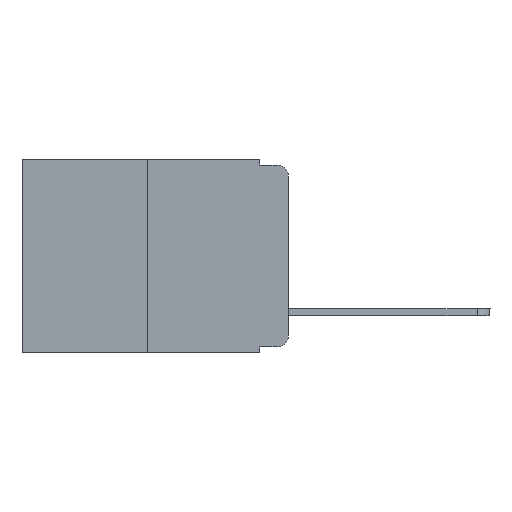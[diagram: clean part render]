
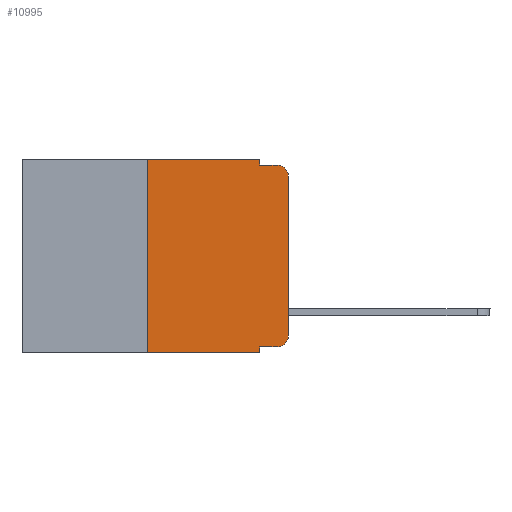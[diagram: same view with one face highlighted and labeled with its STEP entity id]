
A CAD part, left-side view. The second image highlights one B-rep face of the part: STEP entity #10995.
In plain terms, the highlighted planar face has unit normal (-1, 0, 0).
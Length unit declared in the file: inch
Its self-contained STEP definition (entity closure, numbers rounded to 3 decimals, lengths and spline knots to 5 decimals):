
#72 = ORIENTED_EDGE ( 'NONE', *, *, #10749, .T. ) ;
#317 = CARTESIAN_POINT ( 'NONE',  ( 0., 0.051, -0.01 ) ) ;
#686 = CIRCLE ( 'NONE', #3848, 0.02 ) ;
#906 = ORIENTED_EDGE ( 'NONE', *, *, #10365, .T. ) ;
#1024 = CARTESIAN_POINT ( 'NONE',  ( 0., 0.051, -0.01 ) ) ;
#1031 = VECTOR ( 'NONE', #2247, 39.37008 ) ;
#1064 = CARTESIAN_POINT ( 'NONE',  ( 0., 0., -0.313 ) ) ;
#1391 = FACE_OUTER_BOUND ( 'NONE', #3093, .T. ) ;
#1834 = EDGE_CURVE ( 'NONE', #2476, #7793, #9670, .T. ) ;
#1972 = DIRECTION ( 'NONE',  ( 0., 0., 1. ) ) ;
#2091 = CARTESIAN_POINT ( 'NONE',  ( 0., 0.051, -0.333 ) ) ;
#2111 = LINE ( 'NONE', #15091, #1031 ) ;
#2233 = VERTEX_POINT ( 'NONE', #2091 ) ;
#2247 = DIRECTION ( 'NONE',  ( 0., -1., 0. ) ) ;
#2476 = VERTEX_POINT ( 'NONE', #13653 ) ;
#2675 = VECTOR ( 'NONE', #14625, 39.37008 ) ;
#2792 = VERTEX_POINT ( 'NONE', #9612 ) ;
#2924 = DIRECTION ( 'NONE',  ( 0., 0., -1. ) ) ;
#2927 = CARTESIAN_POINT ( 'NONE',  ( 0., 0.473, 0. ) ) ;
#2997 = VERTEX_POINT ( 'NONE', #317 ) ;
#3093 = EDGE_LOOP ( 'NONE', ( #7007, #10981, #4422, #7299, #9044, #7725, #906, #5484, #3766, #72 ) ) ;
#3250 = VECTOR ( 'NONE', #4309, 39.37008 ) ;
#3604 = LINE ( 'NONE', #8515, #3250 ) ;
#3616 = CARTESIAN_POINT ( 'NONE',  ( 0., 0.02, -0.313 ) ) ;
#3766 = ORIENTED_EDGE ( 'NONE', *, *, #14106, .T. ) ;
#3848 = AXIS2_PLACEMENT_3D ( 'NONE', #3616, #11765, #4812 ) ;
#4066 = PLANE ( 'NONE',  #11367 ) ;
#4309 = DIRECTION ( 'NONE',  ( 0., -1., 0. ) ) ;
#4422 = ORIENTED_EDGE ( 'NONE', *, *, #8177, .F. ) ;
#4691 = CARTESIAN_POINT ( 'NONE',  ( 0., 0.25, 0. ) ) ;
#4705 = LINE ( 'NONE', #12380, #2675 ) ;
#4812 = DIRECTION ( 'NONE',  ( 0., 0., -1. ) ) ;
#4843 = EDGE_CURVE ( 'NONE', #2233, #7356, #4705, .T. ) ;
#4847 = CARTESIAN_POINT ( 'NONE',  ( 0., 0.25, 0. ) ) ;
#4967 = VECTOR ( 'NONE', #6954, 39.37008 ) ;
#5444 = CARTESIAN_POINT ( 'NONE',  ( 0., 0.25, -0.343 ) ) ;
#5484 = ORIENTED_EDGE ( 'NONE', *, *, #4843, .F. ) ;
#5911 = LINE ( 'NONE', #7945, #12853 ) ;
#6164 = EDGE_CURVE ( 'NONE', #13422, #2476, #5911, .T. ) ;
#6198 = VERTEX_POINT ( 'NONE', #4691 ) ;
#6243 = CARTESIAN_POINT ( 'NONE',  ( 0., 0.051, 0. ) ) ;
#6444 = DIRECTION ( 'NONE',  ( 1., 0., 0. ) ) ;
#6586 = CARTESIAN_POINT ( 'NONE',  ( 0., 0.02, -0.03 ) ) ;
#6954 = DIRECTION ( 'NONE',  ( 0., -1., 0. ) ) ;
#7007 = ORIENTED_EDGE ( 'NONE', *, *, #6164, .T. ) ;
#7168 = CARTESIAN_POINT ( 'NONE',  ( 0., 0.473, 0. ) ) ;
#7299 = ORIENTED_EDGE ( 'NONE', *, *, #12039, .F. ) ;
#7356 = VERTEX_POINT ( 'NONE', #11218 ) ;
#7725 = ORIENTED_EDGE ( 'NONE', *, *, #12979, .F. ) ;
#7793 = VERTEX_POINT ( 'NONE', #8646 ) ;
#7945 = CARTESIAN_POINT ( 'NONE',  ( 0., 0., 0. ) ) ;
#7950 = VECTOR ( 'NONE', #8451, 39.37008 ) ;
#8177 = EDGE_CURVE ( 'NONE', #2997, #7793, #12072, .T. ) ;
#8451 = DIRECTION ( 'NONE',  ( 0., -1., 0. ) ) ;
#8515 = CARTESIAN_POINT ( 'NONE',  ( 0., 0.473, -0.343 ) ) ;
#8646 = CARTESIAN_POINT ( 'NONE',  ( 0., 0.02, -0.01 ) ) ;
#8687 = DIRECTION ( 'NONE',  ( 0., 0., -1. ) ) ;
#8708 = VECTOR ( 'NONE', #9668, 39.37008 ) ;
#8749 = VERTEX_POINT ( 'NONE', #14119 ) ;
#8968 = DIRECTION ( 'NONE',  ( 0., 0., -1. ) ) ;
#9044 = ORIENTED_EDGE ( 'NONE', *, *, #14207, .F. ) ;
#9561 = LINE ( 'NONE', #7168, #7950 ) ;
#9612 = CARTESIAN_POINT ( 'NONE',  ( 0., 0.051, 0. ) ) ;
#9668 = DIRECTION ( 'NONE',  ( 0., 0., 1. ) ) ;
#9670 = CIRCLE ( 'NONE', #15122, 0.02 ) ;
#10365 = EDGE_CURVE ( 'NONE', #13367, #7356, #3604, .T. ) ;
#10720 = VECTOR ( 'NONE', #2924, 39.37008 ) ;
#10749 = EDGE_CURVE ( 'NONE', #8749, #13422, #686, .T. ) ;
#10981 = ORIENTED_EDGE ( 'NONE', *, *, #1834, .T. ) ;
#10995 = ADVANCED_FACE ( 'NONE', ( #1391 ), #4066, .F. ) ;
#11218 = CARTESIAN_POINT ( 'NONE',  ( 0., 0.051, -0.343 ) ) ;
#11324 = DIRECTION ( 'NONE',  ( -1., 0., 0. ) ) ;
#11367 = AXIS2_PLACEMENT_3D ( 'NONE', #2927, #6444, #8687 ) ;
#11765 = DIRECTION ( 'NONE',  ( -1., 0., 0. ) ) ;
#12021 = LINE ( 'NONE', #6243, #10720 ) ;
#12039 = EDGE_CURVE ( 'NONE', #2792, #2997, #12021, .T. ) ;
#12072 = LINE ( 'NONE', #1024, #4967 ) ;
#12380 = CARTESIAN_POINT ( 'NONE',  ( 0., 0.051, 0. ) ) ;
#12853 = VECTOR ( 'NONE', #1972, 39.37008 ) ;
#12979 = EDGE_CURVE ( 'NONE', #13367, #6198, #14215, .T. ) ;
#13367 = VERTEX_POINT ( 'NONE', #5444 ) ;
#13422 = VERTEX_POINT ( 'NONE', #1064 ) ;
#13653 = CARTESIAN_POINT ( 'NONE',  ( 0., 0., -0.03 ) ) ;
#14106 = EDGE_CURVE ( 'NONE', #2233, #8749, #2111, .T. ) ;
#14119 = CARTESIAN_POINT ( 'NONE',  ( 0., 0.02, -0.333 ) ) ;
#14207 = EDGE_CURVE ( 'NONE', #6198, #2792, #9561, .T. ) ;
#14215 = LINE ( 'NONE', #4847, #8708 ) ;
#14625 = DIRECTION ( 'NONE',  ( 0., 0., -1. ) ) ;
#15091 = CARTESIAN_POINT ( 'NONE',  ( 0., 0.051, -0.333 ) ) ;
#15122 = AXIS2_PLACEMENT_3D ( 'NONE', #6586, #11324, #8968 ) ;
